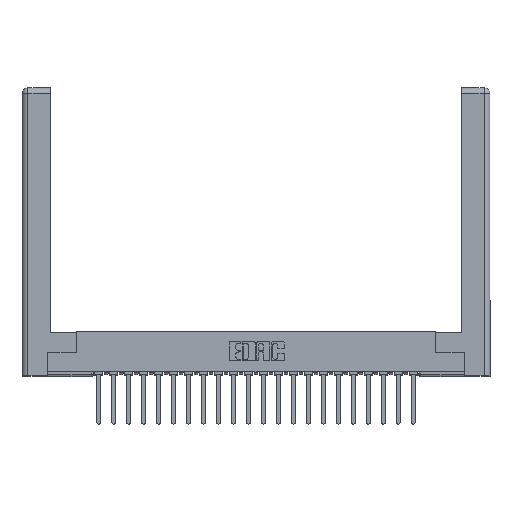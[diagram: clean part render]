
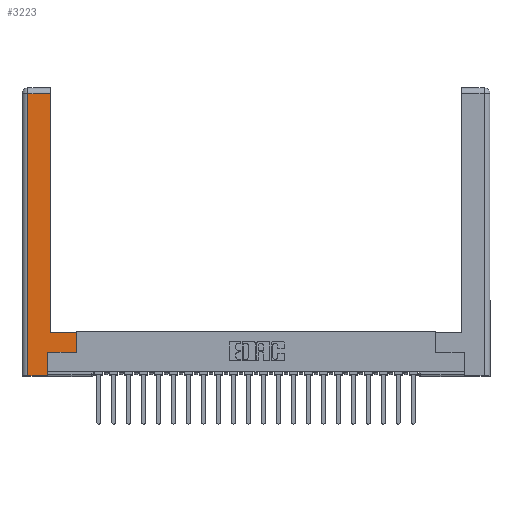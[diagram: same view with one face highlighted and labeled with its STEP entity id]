
A CAD part, top view. The second image highlights one B-rep face of the part: STEP entity #3223.
In plain terms, the highlighted planar face has unit normal (0, 0, 1).
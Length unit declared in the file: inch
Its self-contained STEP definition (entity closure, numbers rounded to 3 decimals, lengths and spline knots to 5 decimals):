
#276 = CARTESIAN_POINT ( 'NONE',  ( 0.0615, 0., 0. ) ) ;
#304 = VERTEX_POINT ( 'NONE', #15923 ) ;
#393 = LINE ( 'NONE', #19211, #2459 ) ;
#1002 = ORIENTED_EDGE ( 'NONE', *, *, #17665, .T. ) ;
#1371 = DIRECTION ( 'NONE',  ( 0., 1., 0. ) ) ;
#1783 = CARTESIAN_POINT ( 'NONE',  ( 0.565, 0.245, 0. ) ) ;
#1822 = ORIENTED_EDGE ( 'NONE', *, *, #21857, .T. ) ;
#2459 = VECTOR ( 'NONE', #8101, 39.37008 ) ;
#2563 = EDGE_CURVE ( 'NONE', #16890, #16938, #393, .T. ) ;
#3084 = VECTOR ( 'NONE', #23237, 39.37008 ) ;
#3223 = ADVANCED_FACE ( 'NONE', ( #21805 ), #13579, .F. ) ;
#3291 = EDGE_LOOP ( 'NONE', ( #1822, #3862, #1002, #12404, #6876, #23260, #19314, #20658 ) ) ;
#3862 = ORIENTED_EDGE ( 'NONE', *, *, #4581, .T. ) ;
#4581 = EDGE_CURVE ( 'NONE', #20304, #19221, #20540, .T. ) ;
#5252 = CARTESIAN_POINT ( 'NONE',  ( 0.265, 0.245, 0. ) ) ;
#5526 = VERTEX_POINT ( 'NONE', #6316 ) ;
#6316 = CARTESIAN_POINT ( 'NONE',  ( 0.565, 0.45, 0. ) ) ;
#6876 = ORIENTED_EDGE ( 'NONE', *, *, #12358, .T. ) ;
#7121 = LINE ( 'NONE', #9847, #15199 ) ;
#7741 = LINE ( 'NONE', #15487, #17287 ) ;
#8101 = DIRECTION ( 'NONE',  ( 1., 0., 0. ) ) ;
#9184 = LINE ( 'NONE', #10552, #22020 ) ;
#9847 = CARTESIAN_POINT ( 'NONE',  ( 0.265, 0., 0. ) ) ;
#10391 = VERTEX_POINT ( 'NONE', #10944 ) ;
#10552 = CARTESIAN_POINT ( 'NONE',  ( 0.565, 0.45, 0. ) ) ;
#10944 = CARTESIAN_POINT ( 'NONE',  ( 0.0615, 0., 0. ) ) ;
#11013 = LINE ( 'NONE', #12791, #12510 ) ;
#12358 = EDGE_CURVE ( 'NONE', #14322, #16890, #11013, .T. ) ;
#12404 = ORIENTED_EDGE ( 'NONE', *, *, #12541, .T. ) ;
#12510 = VECTOR ( 'NONE', #1371, 39.37008 ) ;
#12541 = EDGE_CURVE ( 'NONE', #10391, #14322, #7121, .T. ) ;
#12564 = DIRECTION ( 'NONE',  ( 0., 1., 0. ) ) ;
#12791 = CARTESIAN_POINT ( 'NONE',  ( 0.265, 0.245, 0. ) ) ;
#13579 = PLANE ( 'NONE',  #20887 ) ;
#14322 = VERTEX_POINT ( 'NONE', #15191 ) ;
#15191 = CARTESIAN_POINT ( 'NONE',  ( 0.265, 0., 0. ) ) ;
#15199 = VECTOR ( 'NONE', #17440, 39.37008 ) ;
#15301 = EDGE_CURVE ( 'NONE', #16938, #5526, #9184, .T. ) ;
#15487 = CARTESIAN_POINT ( 'NONE',  ( 0.295, 0.45, 0. ) ) ;
#15489 = CARTESIAN_POINT ( 'NONE',  ( 0., 0., 0. ) ) ;
#15744 = DIRECTION ( 'NONE',  ( -1., 0., 0. ) ) ;
#15923 = CARTESIAN_POINT ( 'NONE',  ( 0.295, 0.45, 0. ) ) ;
#16023 = CARTESIAN_POINT ( 'NONE',  ( 0.295, 2.94, 0. ) ) ;
#16152 = CARTESIAN_POINT ( 'NONE',  ( 0.0615, 2.94, 0. ) ) ;
#16674 = VECTOR ( 'NONE', #24101, 39.37008 ) ;
#16841 = VECTOR ( 'NONE', #22161, 39.37008 ) ;
#16890 = VERTEX_POINT ( 'NONE', #5252 ) ;
#16938 = VERTEX_POINT ( 'NONE', #1783 ) ;
#17287 = VECTOR ( 'NONE', #24656, 39.37008 ) ;
#17405 = DIRECTION ( 'NONE',  ( 0., 0., -1. ) ) ;
#17440 = DIRECTION ( 'NONE',  ( 1., 0., 0. ) ) ;
#17665 = EDGE_CURVE ( 'NONE', #19221, #10391, #24579, .T. ) ;
#19211 = CARTESIAN_POINT ( 'NONE',  ( 0.565, 0.245, 0. ) ) ;
#19221 = VERTEX_POINT ( 'NONE', #16152 ) ;
#19314 = ORIENTED_EDGE ( 'NONE', *, *, #15301, .T. ) ;
#20304 = VERTEX_POINT ( 'NONE', #16023 ) ;
#20463 = CARTESIAN_POINT ( 'NONE',  ( 0.0615, 2.94, 0. ) ) ;
#20540 = LINE ( 'NONE', #20463, #16674 ) ;
#20658 = ORIENTED_EDGE ( 'NONE', *, *, #20751, .T. ) ;
#20751 = EDGE_CURVE ( 'NONE', #5526, #304, #7741, .T. ) ;
#20887 = AXIS2_PLACEMENT_3D ( 'NONE', #15489, #17405, #15744 ) ;
#21805 = FACE_OUTER_BOUND ( 'NONE', #3291, .T. ) ;
#21857 = EDGE_CURVE ( 'NONE', #304, #20304, #21902, .T. ) ;
#21902 = LINE ( 'NONE', #24373, #16841 ) ;
#22020 = VECTOR ( 'NONE', #12564, 39.37008 ) ;
#22161 = DIRECTION ( 'NONE',  ( 0., 1., 0. ) ) ;
#23237 = DIRECTION ( 'NONE',  ( 0., -1., 0. ) ) ;
#23260 = ORIENTED_EDGE ( 'NONE', *, *, #2563, .T. ) ;
#24101 = DIRECTION ( 'NONE',  ( -1., 0., 0. ) ) ;
#24373 = CARTESIAN_POINT ( 'NONE',  ( 0.295, 3., 0. ) ) ;
#24579 = LINE ( 'NONE', #276, #3084 ) ;
#24656 = DIRECTION ( 'NONE',  ( -1., 0., 0. ) ) ;
